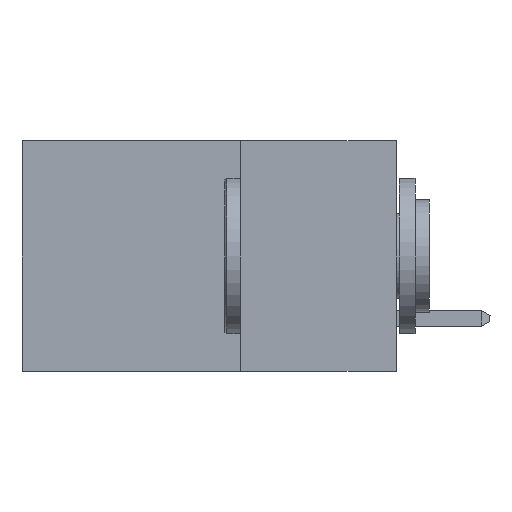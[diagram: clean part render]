
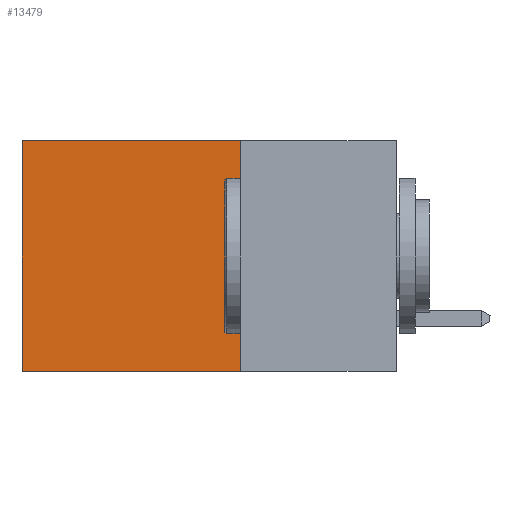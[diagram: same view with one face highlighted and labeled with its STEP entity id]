
A CAD part, left-side view. The second image highlights one B-rep face of the part: STEP entity #13479.
In plain terms, the highlighted planar face has unit normal (-1, 0, 0).
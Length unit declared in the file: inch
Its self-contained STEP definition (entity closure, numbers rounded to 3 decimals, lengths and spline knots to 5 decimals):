
#749 = CARTESIAN_POINT ( 'NONE',  ( 0.2615, 0.25, -0.37 ) ) ;
#1102 = CARTESIAN_POINT ( 'NONE',  ( 0.2615, 0.25, -0.37 ) ) ;
#1308 = VERTEX_POINT ( 'NONE', #5492 ) ;
#1362 = VERTEX_POINT ( 'NONE', #7251 ) ;
#1841 = PLANE ( 'NONE',  #3201 ) ;
#2919 = DIRECTION ( 'NONE',  ( 0., 0., -1. ) ) ;
#3081 = LINE ( 'NONE', #10180, #13388 ) ;
#3201 = AXIS2_PLACEMENT_3D ( 'NONE', #749, #9314, #2919 ) ;
#3334 = EDGE_CURVE ( 'NONE', #7509, #1308, #10037, .T. ) ;
#3435 = ORIENTED_EDGE ( 'NONE', *, *, #10634, .F. ) ;
#3449 = VECTOR ( 'NONE', #8312, 39.37008 ) ;
#3563 = EDGE_LOOP ( 'NONE', ( #8232, #3435, #8567, #10877 ) ) ;
#4113 = LINE ( 'NONE', #4779, #9423 ) ;
#4779 = CARTESIAN_POINT ( 'NONE',  ( 0.2615, 0.25, 0. ) ) ;
#4835 = CARTESIAN_POINT ( 'NONE',  ( 0.2615, 0.25, 0. ) ) ;
#5492 = CARTESIAN_POINT ( 'NONE',  ( 0.2615, 0.25, -0.37 ) ) ;
#5858 = DIRECTION ( 'NONE',  ( 0., 1., 0. ) ) ;
#5998 = DIRECTION ( 'NONE',  ( 0., 0., -1. ) ) ;
#7048 = CARTESIAN_POINT ( 'NONE',  ( 0.2615, 0.6, 0. ) ) ;
#7251 = CARTESIAN_POINT ( 'NONE',  ( 0.2615, 0.6, -0.37 ) ) ;
#7254 = CARTESIAN_POINT ( 'NONE',  ( 0.2615, 0.25, -0.37 ) ) ;
#7509 = VERTEX_POINT ( 'NONE', #4835 ) ;
#8232 = ORIENTED_EDGE ( 'NONE', *, *, #11225, .T. ) ;
#8312 = DIRECTION ( 'NONE',  ( 0., 1., 0. ) ) ;
#8567 = ORIENTED_EDGE ( 'NONE', *, *, #3334, .F. ) ;
#8846 = DIRECTION ( 'NONE',  ( 0., 0., -1. ) ) ;
#9314 = DIRECTION ( 'NONE',  ( 1., 0., 0. ) ) ;
#9423 = VECTOR ( 'NONE', #5858, 39.37008 ) ;
#9432 = LINE ( 'NONE', #7254, #3449 ) ;
#9517 = FACE_OUTER_BOUND ( 'NONE', #3563, .T. ) ;
#10037 = LINE ( 'NONE', #1102, #12544 ) ;
#10180 = CARTESIAN_POINT ( 'NONE',  ( 0.2615, 0.6, -0.37 ) ) ;
#10634 = EDGE_CURVE ( 'NONE', #1308, #1362, #9432, .T. ) ;
#10877 = ORIENTED_EDGE ( 'NONE', *, *, #11108, .T. ) ;
#11108 = EDGE_CURVE ( 'NONE', #7509, #11617, #4113, .T. ) ;
#11225 = EDGE_CURVE ( 'NONE', #11617, #1362, #3081, .T. ) ;
#11617 = VERTEX_POINT ( 'NONE', #7048 ) ;
#12544 = VECTOR ( 'NONE', #8846, 39.37008 ) ;
#13388 = VECTOR ( 'NONE', #5998, 39.37008 ) ;
#13479 = ADVANCED_FACE ( 'NONE', ( #9517 ), #1841, .F. ) ;
